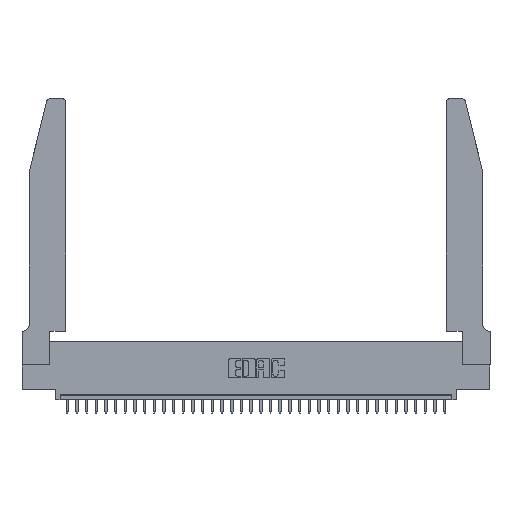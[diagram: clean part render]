
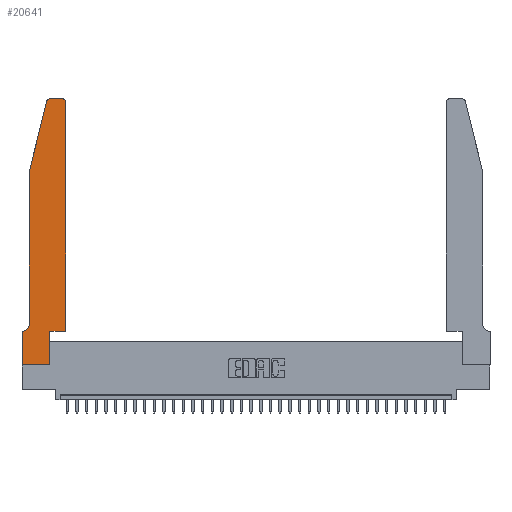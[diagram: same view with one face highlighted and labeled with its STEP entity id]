
A CAD part, top view. The second image highlights one B-rep face of the part: STEP entity #20641.
In plain terms, the highlighted planar face has unit normal (0, 0, 1).
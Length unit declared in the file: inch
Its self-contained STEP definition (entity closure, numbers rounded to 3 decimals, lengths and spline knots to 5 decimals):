
#136 = CIRCLE ( 'NONE', #23951, 0.07 ) ;
#140 = DIRECTION ( 'NONE',  ( -1., 0., 0. ) ) ;
#147 = ORIENTED_EDGE ( 'NONE', *, *, #30745, .T. ) ;
#234 = LINE ( 'NONE', #31368, #20288 ) ;
#343 = DIRECTION ( 'NONE',  ( 1., 0., 0. ) ) ;
#392 = LINE ( 'NONE', #26325, #27654 ) ;
#499 = VERTEX_POINT ( 'NONE', #16490 ) ;
#661 = VERTEX_POINT ( 'NONE', #6269 ) ;
#1759 = LINE ( 'NONE', #19593, #13224 ) ;
#2232 = ORIENTED_EDGE ( 'NONE', *, *, #9807, .T. ) ;
#2347 = DIRECTION ( 'NONE',  ( 0., 1., 0. ) ) ;
#3107 = VERTEX_POINT ( 'NONE', #16370 ) ;
#4038 = AXIS2_PLACEMENT_3D ( 'NONE', #19711, #22249, #33197 ) ;
#4091 = DIRECTION ( 'NONE',  ( -1., 0., 0. ) ) ;
#4106 = LINE ( 'NONE', #6694, #33912 ) ;
#4247 = DIRECTION ( 'NONE',  ( 0., 1., 0. ) ) ;
#4286 = ORIENTED_EDGE ( 'NONE', *, *, #23257, .T. ) ;
#4598 = EDGE_LOOP ( 'NONE', ( #14453, #28133, #14388, #13555, #14833, #5268, #28791, #2232, #147, #4286, #9120, #16064 ) ) ;
#5268 = ORIENTED_EDGE ( 'NONE', *, *, #12497, .T. ) ;
#6269 = CARTESIAN_POINT ( 'NONE',  ( 0.0755, 0.42, 0.37 ) ) ;
#6438 = VERTEX_POINT ( 'NONE', #18874 ) ;
#6694 = CARTESIAN_POINT ( 'NONE',  ( 0.4505, 0.35, 0.37 ) ) ;
#6698 = CIRCLE ( 'NONE', #14528, 0.03 ) ;
#7507 = CARTESIAN_POINT ( 'NONE',  ( 0., 0., 0.37 ) ) ;
#7767 = VECTOR ( 'NONE', #4247, 39.37008 ) ;
#8310 = DIRECTION ( 'NONE',  ( 0., -1., 0. ) ) ;
#8341 = VERTEX_POINT ( 'NONE', #12747 ) ;
#9120 = ORIENTED_EDGE ( 'NONE', *, *, #12426, .T. ) ;
#9807 = EDGE_CURVE ( 'NONE', #27349, #31481, #11065, .T. ) ;
#10099 = VERTEX_POINT ( 'NONE', #13021 ) ;
#10641 = VECTOR ( 'NONE', #31373, 39.37008 ) ;
#11065 = LINE ( 'NONE', #28839, #10641 ) ;
#12030 = VERTEX_POINT ( 'NONE', #23903 ) ;
#12426 = EDGE_CURVE ( 'NONE', #31147, #499, #4106, .T. ) ;
#12497 = EDGE_CURVE ( 'NONE', #12030, #6438, #234, .T. ) ;
#12747 = CARTESIAN_POINT ( 'NONE',  ( 0.0755, 2., 0.37 ) ) ;
#13021 = CARTESIAN_POINT ( 'NONE',  ( 0.2865, 0.35, 0.37 ) ) ;
#13224 = VECTOR ( 'NONE', #8310, 39.37008 ) ;
#13555 = ORIENTED_EDGE ( 'NONE', *, *, #20714, .T. ) ;
#13567 = CARTESIAN_POINT ( 'NONE',  ( 0.0055, 0.42, 0.37 ) ) ;
#13645 = CARTESIAN_POINT ( 'NONE',  ( 0.4205, 2.72, 0.37 ) ) ;
#14388 = ORIENTED_EDGE ( 'NONE', *, *, #25946, .T. ) ;
#14453 = ORIENTED_EDGE ( 'NONE', *, *, #19753, .T. ) ;
#14528 = AXIS2_PLACEMENT_3D ( 'NONE', #13645, #32988, #343 ) ;
#14833 = ORIENTED_EDGE ( 'NONE', *, *, #25523, .T. ) ;
#14846 = VECTOR ( 'NONE', #16622, 39.37008 ) ;
#15039 = LINE ( 'NONE', #23150, #24805 ) ;
#16064 = ORIENTED_EDGE ( 'NONE', *, *, #24293, .T. ) ;
#16068 = EDGE_CURVE ( 'NONE', #29371, #26870, #29757, .T. ) ;
#16370 = CARTESIAN_POINT ( 'NONE',  ( 0.4205, 2.75, 0.37 ) ) ;
#16490 = CARTESIAN_POINT ( 'NONE',  ( 0.4505, 2.72, 0.37 ) ) ;
#16499 = CARTESIAN_POINT ( 'NONE',  ( 0.4505, 0.35, 0.37 ) ) ;
#16622 = DIRECTION ( 'NONE',  ( 1., 0., 0. ) ) ;
#16851 = LINE ( 'NONE', #7507, #22436 ) ;
#17778 = CARTESIAN_POINT ( 'NONE',  ( 0.2865, 0.35, 0.37 ) ) ;
#17984 = EDGE_CURVE ( 'NONE', #6438, #27349, #16851, .T. ) ;
#18219 = DIRECTION ( 'NONE',  ( -0.239, -0.971, 0. ) ) ;
#18324 = DIRECTION ( 'NONE',  ( 1., 0., 0. ) ) ;
#18874 = CARTESIAN_POINT ( 'NONE',  ( 0., 0.35, 0.37 ) ) ;
#19593 = CARTESIAN_POINT ( 'NONE',  ( 0.0755, 2., 0.37 ) ) ;
#19711 = CARTESIAN_POINT ( 'NONE',  ( 0.284, 2.72, 0.37 ) ) ;
#19753 = EDGE_CURVE ( 'NONE', #3107, #29371, #15039, .T. ) ;
#20288 = VECTOR ( 'NONE', #23665, 39.37008 ) ;
#20641 = ADVANCED_FACE ( 'NONE', ( #32863 ), #32146, .T. ) ;
#20714 = EDGE_CURVE ( 'NONE', #8341, #661, #1759, .T. ) ;
#21714 = DIRECTION ( 'NONE',  ( 0., 0., -1. ) ) ;
#22071 = LINE ( 'NONE', #16499, #14846 ) ;
#22249 = DIRECTION ( 'NONE',  ( 0., 0., 1. ) ) ;
#22436 = VECTOR ( 'NONE', #32631, 39.37008 ) ;
#23126 = LINE ( 'NONE', #17778, #7767 ) ;
#23150 = CARTESIAN_POINT ( 'NONE',  ( 0.2605, 2.75, 0.37 ) ) ;
#23257 = EDGE_CURVE ( 'NONE', #10099, #31147, #22071, .T. ) ;
#23665 = DIRECTION ( 'NONE',  ( -1., 0., 0. ) ) ;
#23903 = CARTESIAN_POINT ( 'NONE',  ( 0.0055, 0.35, 0.37 ) ) ;
#23951 = AXIS2_PLACEMENT_3D ( 'NONE', #13567, #21714, #140 ) ;
#24133 = CARTESIAN_POINT ( 'NONE',  ( 0., 0., 0.37 ) ) ;
#24293 = EDGE_CURVE ( 'NONE', #499, #3107, #6698, .T. ) ;
#24657 = CARTESIAN_POINT ( 'NONE',  ( 0.4505, 0.35, 0.37 ) ) ;
#24805 = VECTOR ( 'NONE', #4091, 39.37008 ) ;
#25523 = EDGE_CURVE ( 'NONE', #661, #12030, #136, .T. ) ;
#25946 = EDGE_CURVE ( 'NONE', #26870, #8341, #392, .T. ) ;
#26325 = CARTESIAN_POINT ( 'NONE',  ( 0.0755, 2., 0.37 ) ) ;
#26870 = VERTEX_POINT ( 'NONE', #32749 ) ;
#27349 = VERTEX_POINT ( 'NONE', #24133 ) ;
#27654 = VECTOR ( 'NONE', #18219, 39.37008 ) ;
#27868 = CARTESIAN_POINT ( 'NONE',  ( 0.284, 2.75, 0.37 ) ) ;
#27895 = CARTESIAN_POINT ( 'NONE',  ( 0., 0.35, 0.37 ) ) ;
#28133 = ORIENTED_EDGE ( 'NONE', *, *, #16068, .T. ) ;
#28791 = ORIENTED_EDGE ( 'NONE', *, *, #17984, .T. ) ;
#28839 = CARTESIAN_POINT ( 'NONE',  ( 0., 0., 0.37 ) ) ;
#29371 = VERTEX_POINT ( 'NONE', #27868 ) ;
#29757 = CIRCLE ( 'NONE', #4038, 0.03 ) ;
#30745 = EDGE_CURVE ( 'NONE', #31481, #10099, #23126, .T. ) ;
#31147 = VERTEX_POINT ( 'NONE', #24657 ) ;
#31368 = CARTESIAN_POINT ( 'NONE',  ( 0.0755, 0.35, 0.37 ) ) ;
#31373 = DIRECTION ( 'NONE',  ( 1., 0., 0. ) ) ;
#31481 = VERTEX_POINT ( 'NONE', #31834 ) ;
#31834 = CARTESIAN_POINT ( 'NONE',  ( 0.2865, 0., 0.37 ) ) ;
#31960 = AXIS2_PLACEMENT_3D ( 'NONE', #27895, #32772, #18324 ) ;
#32146 = PLANE ( 'NONE',  #31960 ) ;
#32631 = DIRECTION ( 'NONE',  ( 0., -1., 0. ) ) ;
#32749 = CARTESIAN_POINT ( 'NONE',  ( 0.25487, 2.72718, 0.37 ) ) ;
#32772 = DIRECTION ( 'NONE',  ( 0., 0., 1. ) ) ;
#32863 = FACE_OUTER_BOUND ( 'NONE', #4598, .T. ) ;
#32988 = DIRECTION ( 'NONE',  ( 0., 0., 1. ) ) ;
#33197 = DIRECTION ( 'NONE',  ( 1., 0., 0. ) ) ;
#33912 = VECTOR ( 'NONE', #2347, 39.37008 ) ;
